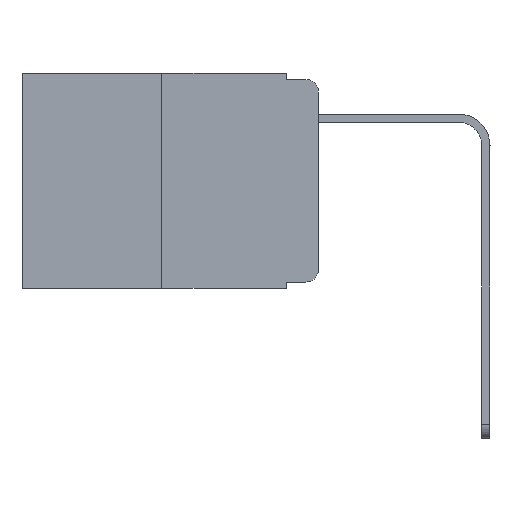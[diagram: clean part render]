
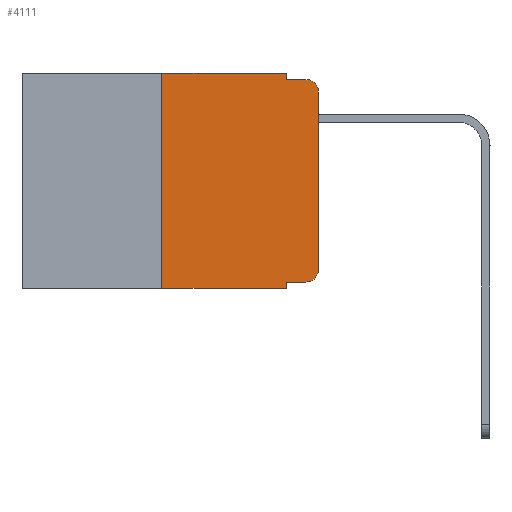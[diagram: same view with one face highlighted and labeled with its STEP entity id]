
A CAD part, left-side view. The second image highlights one B-rep face of the part: STEP entity #4111.
In plain terms, the highlighted planar face has unit normal (-1, 0, 0).
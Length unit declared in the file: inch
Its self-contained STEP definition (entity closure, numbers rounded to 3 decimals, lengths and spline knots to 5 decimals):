
#27 = CARTESIAN_POINT ( 'NONE',  ( 0., 0.051, -0.333 ) ) ;
#234 = VERTEX_POINT ( 'NONE', #1120 ) ;
#291 = AXIS2_PLACEMENT_3D ( 'NONE', #19009, #1481, #20595 ) ;
#452 = CARTESIAN_POINT ( 'NONE',  ( 0., 0.051, -0.01 ) ) ;
#642 = LINE ( 'NONE', #19025, #4418 ) ;
#1120 = CARTESIAN_POINT ( 'NONE',  ( 0., 0.02, -0.01 ) ) ;
#1353 = DIRECTION ( 'NONE',  ( 0., -1., 0. ) ) ;
#1384 = DIRECTION ( 'NONE',  ( 0., 0., 1. ) ) ;
#1481 = DIRECTION ( 'NONE',  ( 1., 0., 0. ) ) ;
#1627 = LINE ( 'NONE', #16376, #5169 ) ;
#1727 = VERTEX_POINT ( 'NONE', #6609 ) ;
#1767 = DIRECTION ( 'NONE',  ( 0., -1., 0. ) ) ;
#1986 = EDGE_CURVE ( 'NONE', #11670, #16834, #20690, .T. ) ;
#2329 = CARTESIAN_POINT ( 'NONE',  ( 0., 0.02, -0.313 ) ) ;
#2337 = LINE ( 'NONE', #7098, #9391 ) ;
#2582 = VECTOR ( 'NONE', #5395, 39.37008 ) ;
#3301 = DIRECTION ( 'NONE',  ( 0., 0., -1. ) ) ;
#3305 = CARTESIAN_POINT ( 'NONE',  ( 0., 0.051, -0.01 ) ) ;
#3322 = EDGE_CURVE ( 'NONE', #3621, #18097, #12188, .T. ) ;
#3359 = PLANE ( 'NONE',  #291 ) ;
#3531 = VERTEX_POINT ( 'NONE', #452 ) ;
#3621 = VERTEX_POINT ( 'NONE', #11594 ) ;
#3678 = VECTOR ( 'NONE', #1384, 39.37008 ) ;
#3887 = CARTESIAN_POINT ( 'NONE',  ( 0., 0.051, -0.333 ) ) ;
#3972 = DIRECTION ( 'NONE',  ( -1., 0., 0. ) ) ;
#4111 = ADVANCED_FACE ( 'NONE', ( #11651 ), #3359, .F. ) ;
#4418 = VECTOR ( 'NONE', #1353, 39.37008 ) ;
#4688 = EDGE_CURVE ( 'NONE', #19738, #16671, #18606, .T. ) ;
#5169 = VECTOR ( 'NONE', #8451, 39.37008 ) ;
#5183 = CARTESIAN_POINT ( 'NONE',  ( 0., 0.25, 0. ) ) ;
#5395 = DIRECTION ( 'NONE',  ( 0., 0., 1. ) ) ;
#5591 = DIRECTION ( 'NONE',  ( 0., -1., 0. ) ) ;
#5645 = AXIS2_PLACEMENT_3D ( 'NONE', #2329, #3972, #16898 ) ;
#5761 = CARTESIAN_POINT ( 'NONE',  ( 0., 0.02, -0.333 ) ) ;
#6177 = VECTOR ( 'NONE', #3301, 39.37008 ) ;
#6609 = CARTESIAN_POINT ( 'NONE',  ( 0., 0.051, -0.343 ) ) ;
#7098 = CARTESIAN_POINT ( 'NONE',  ( 0., 0.051, 0. ) ) ;
#7157 = LINE ( 'NONE', #3305, #12613 ) ;
#8037 = EDGE_CURVE ( 'NONE', #16013, #3531, #2337, .T. ) ;
#8346 = CIRCLE ( 'NONE', #14856, 0.02 ) ;
#8451 = DIRECTION ( 'NONE',  ( 0., -1., 0. ) ) ;
#8825 = DIRECTION ( 'NONE',  ( 0., 0., -1. ) ) ;
#8915 = EDGE_CURVE ( 'NONE', #16834, #3621, #9836, .T. ) ;
#9378 = ORIENTED_EDGE ( 'NONE', *, *, #8037, .F. ) ;
#9391 = VECTOR ( 'NONE', #8825, 39.37008 ) ;
#9425 = ORIENTED_EDGE ( 'NONE', *, *, #4688, .F. ) ;
#9658 = ORIENTED_EDGE ( 'NONE', *, *, #19735, .F. ) ;
#9794 = ORIENTED_EDGE ( 'NONE', *, *, #13704, .T. ) ;
#9836 = CIRCLE ( 'NONE', #5645, 0.02 ) ;
#9875 = EDGE_CURVE ( 'NONE', #18097, #234, #8346, .T. ) ;
#9884 = CARTESIAN_POINT ( 'NONE',  ( 0., 0.051, 0. ) ) ;
#10248 = EDGE_LOOP ( 'NONE', ( #12260, #17796, #15644, #9378, #9658, #9425, #9794, #17712, #10583, #14072 ) ) ;
#10583 = ORIENTED_EDGE ( 'NONE', *, *, #1986, .T. ) ;
#10670 = LINE ( 'NONE', #9884, #6177 ) ;
#10988 = CARTESIAN_POINT ( 'NONE',  ( 0., 0.02, -0.03 ) ) ;
#11594 = CARTESIAN_POINT ( 'NONE',  ( 0., 0., -0.313 ) ) ;
#11651 = FACE_OUTER_BOUND ( 'NONE', #10248, .T. ) ;
#11670 = VERTEX_POINT ( 'NONE', #27 ) ;
#11776 = CARTESIAN_POINT ( 'NONE',  ( 0., 0.25, 0. ) ) ;
#12188 = LINE ( 'NONE', #17334, #3678 ) ;
#12227 = VECTOR ( 'NONE', #5591, 39.37008 ) ;
#12260 = ORIENTED_EDGE ( 'NONE', *, *, #3322, .T. ) ;
#12613 = VECTOR ( 'NONE', #1767, 39.37008 ) ;
#13700 = CARTESIAN_POINT ( 'NONE',  ( 0., 0., -0.03 ) ) ;
#13704 = EDGE_CURVE ( 'NONE', #19738, #1727, #1627, .T. ) ;
#14072 = ORIENTED_EDGE ( 'NONE', *, *, #8915, .T. ) ;
#14189 = DIRECTION ( 'NONE',  ( -1., 0., 0. ) ) ;
#14262 = EDGE_CURVE ( 'NONE', #3531, #234, #7157, .T. ) ;
#14856 = AXIS2_PLACEMENT_3D ( 'NONE', #10988, #14189, #17469 ) ;
#15644 = ORIENTED_EDGE ( 'NONE', *, *, #14262, .F. ) ;
#16013 = VERTEX_POINT ( 'NONE', #20681 ) ;
#16376 = CARTESIAN_POINT ( 'NONE',  ( 0., 0.473, -0.343 ) ) ;
#16671 = VERTEX_POINT ( 'NONE', #11776 ) ;
#16834 = VERTEX_POINT ( 'NONE', #5761 ) ;
#16898 = DIRECTION ( 'NONE',  ( 0., 0., -1. ) ) ;
#17334 = CARTESIAN_POINT ( 'NONE',  ( 0., 0., 0. ) ) ;
#17469 = DIRECTION ( 'NONE',  ( 0., 0., -1. ) ) ;
#17500 = CARTESIAN_POINT ( 'NONE',  ( 0., 0.25, -0.343 ) ) ;
#17712 = ORIENTED_EDGE ( 'NONE', *, *, #19901, .F. ) ;
#17796 = ORIENTED_EDGE ( 'NONE', *, *, #9875, .T. ) ;
#18097 = VERTEX_POINT ( 'NONE', #13700 ) ;
#18606 = LINE ( 'NONE', #5183, #2582 ) ;
#19009 = CARTESIAN_POINT ( 'NONE',  ( 0., 0.473, 0. ) ) ;
#19025 = CARTESIAN_POINT ( 'NONE',  ( 0., 0.473, 0. ) ) ;
#19735 = EDGE_CURVE ( 'NONE', #16671, #16013, #642, .T. ) ;
#19738 = VERTEX_POINT ( 'NONE', #17500 ) ;
#19901 = EDGE_CURVE ( 'NONE', #11670, #1727, #10670, .T. ) ;
#20595 = DIRECTION ( 'NONE',  ( 0., 0., -1. ) ) ;
#20681 = CARTESIAN_POINT ( 'NONE',  ( 0., 0.051, 0. ) ) ;
#20690 = LINE ( 'NONE', #3887, #12227 ) ;
